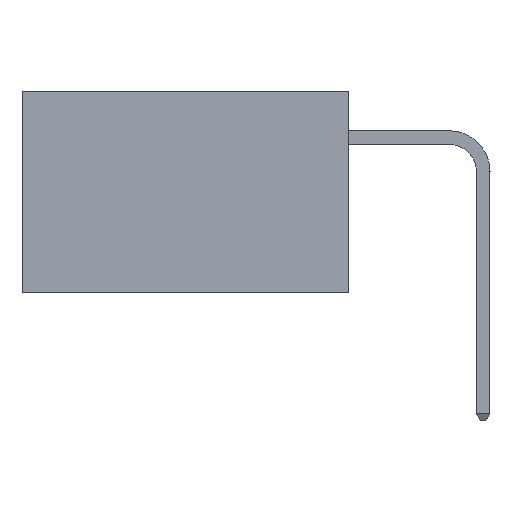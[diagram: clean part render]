
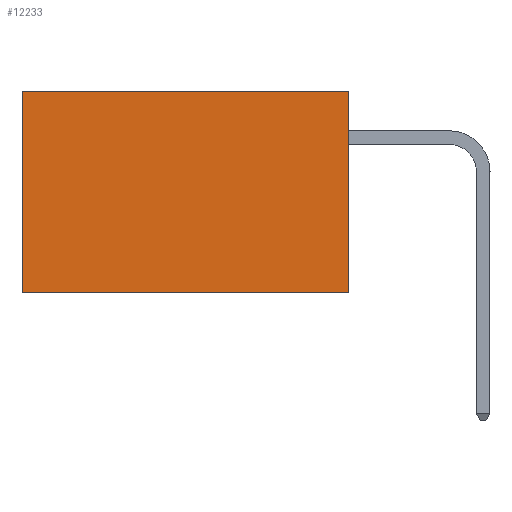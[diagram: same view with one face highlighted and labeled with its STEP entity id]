
A CAD part, left-side view. The second image highlights one B-rep face of the part: STEP entity #12233.
In plain terms, the highlighted planar face has unit normal (-1, 0, 0).
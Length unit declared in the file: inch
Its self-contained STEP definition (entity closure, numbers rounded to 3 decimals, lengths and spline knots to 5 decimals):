
#152 = VERTEX_POINT ( 'NONE', #30437 ) ;
#1678 = ORIENTED_EDGE ( 'NONE', *, *, #6598, .T. ) ;
#2903 = ORIENTED_EDGE ( 'NONE', *, *, #23107, .F. ) ;
#4798 = VERTEX_POINT ( 'NONE', #18086 ) ;
#6277 = EDGE_LOOP ( 'NONE', ( #1678, #2903, #11315, #16597 ) ) ;
#6598 = EDGE_CURVE ( 'NONE', #4798, #19650, #33866, .T. ) ;
#6611 = DIRECTION ( 'NONE',  ( 0., 1., 0. ) ) ;
#7888 = DIRECTION ( 'NONE',  ( 0., 0., -1. ) ) ;
#8487 = CARTESIAN_POINT ( 'NONE',  ( 0.2875, 0.6, 0. ) ) ;
#11315 = ORIENTED_EDGE ( 'NONE', *, *, #31685, .F. ) ;
#12107 = EDGE_CURVE ( 'NONE', #152, #4798, #26906, .T. ) ;
#12233 = ADVANCED_FACE ( 'NONE', ( #26230 ), #16222, .F. ) ;
#15083 = VECTOR ( 'NONE', #29229, 39.37008 ) ;
#15110 = LINE ( 'NONE', #31924, #15083 ) ;
#15188 = DIRECTION ( 'NONE',  ( 0., 0., -1. ) ) ;
#15750 = DIRECTION ( 'NONE',  ( 1., 0., 0. ) ) ;
#16077 = CARTESIAN_POINT ( 'NONE',  ( 0.2875, 0., 0. ) ) ;
#16222 = PLANE ( 'NONE',  #25852 ) ;
#16597 = ORIENTED_EDGE ( 'NONE', *, *, #12107, .T. ) ;
#18086 = CARTESIAN_POINT ( 'NONE',  ( 0.2875, 0.6, 0. ) ) ;
#19650 = VERTEX_POINT ( 'NONE', #19812 ) ;
#19812 = CARTESIAN_POINT ( 'NONE',  ( 0.2875, 0.6, -0.37 ) ) ;
#20372 = VERTEX_POINT ( 'NONE', #31472 ) ;
#22838 = CARTESIAN_POINT ( 'NONE',  ( 0.2875, 0., -0.37 ) ) ;
#23107 = EDGE_CURVE ( 'NONE', #20372, #19650, #25567, .T. ) ;
#25567 = LINE ( 'NONE', #22838, #26034 ) ;
#25852 = AXIS2_PLACEMENT_3D ( 'NONE', #16077, #15750, #15188 ) ;
#26034 = VECTOR ( 'NONE', #6611, 39.37008 ) ;
#26230 = FACE_OUTER_BOUND ( 'NONE', #6277, .T. ) ;
#26906 = LINE ( 'NONE', #32678, #26968 ) ;
#26968 = VECTOR ( 'NONE', #32508, 39.37008 ) ;
#29229 = DIRECTION ( 'NONE',  ( 0., 0., -1. ) ) ;
#30437 = CARTESIAN_POINT ( 'NONE',  ( 0.2875, 0., 0. ) ) ;
#31472 = CARTESIAN_POINT ( 'NONE',  ( 0.2875, 0., -0.37 ) ) ;
#31685 = EDGE_CURVE ( 'NONE', #152, #20372, #15110, .T. ) ;
#31924 = CARTESIAN_POINT ( 'NONE',  ( 0.2875, 0., 0. ) ) ;
#32508 = DIRECTION ( 'NONE',  ( 0., 1., 0. ) ) ;
#32678 = CARTESIAN_POINT ( 'NONE',  ( 0.2875, 0., 0. ) ) ;
#33866 = LINE ( 'NONE', #8487, #34117 ) ;
#34117 = VECTOR ( 'NONE', #7888, 39.37008 ) ;
